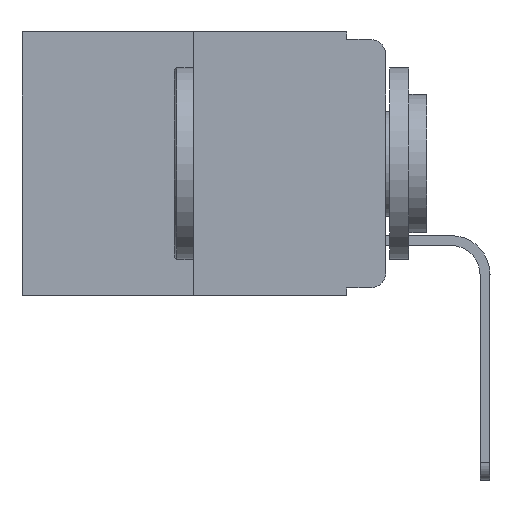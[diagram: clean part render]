
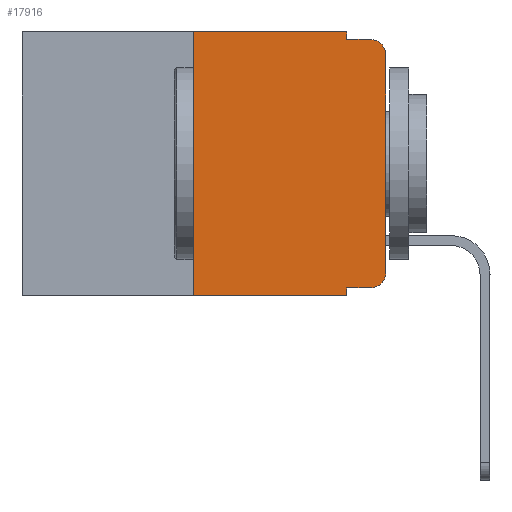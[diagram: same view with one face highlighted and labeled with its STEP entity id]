
A CAD part, left-side view. The second image highlights one B-rep face of the part: STEP entity #17916.
In plain terms, the highlighted planar face has unit normal (-1, 0, 0).
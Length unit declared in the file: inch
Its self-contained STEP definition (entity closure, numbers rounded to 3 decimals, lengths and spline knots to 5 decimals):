
#12 = CARTESIAN_POINT ( 'NONE',  ( 0., 0.051, 0. ) ) ;
#140 = DIRECTION ( 'NONE',  ( 1., 0., 0. ) ) ;
#257 = ORIENTED_EDGE ( 'NONE', *, *, #9310, .T. ) ;
#658 = EDGE_LOOP ( 'NONE', ( #20941, #257, #15732, #19808, #21544, #19864, #11440, #20858, #4094, #17182 ) ) ;
#941 = CIRCLE ( 'NONE', #20716, 0.02 ) ;
#1385 = CARTESIAN_POINT ( 'NONE',  ( 0., 0.25, 0. ) ) ;
#1411 = EDGE_CURVE ( 'NONE', #12307, #14423, #21536, .T. ) ;
#1836 = LINE ( 'NONE', #6421, #13147 ) ;
#2002 = CARTESIAN_POINT ( 'NONE',  ( 0., 0.051, 0. ) ) ;
#2283 = VERTEX_POINT ( 'NONE', #21336 ) ;
#2527 = VECTOR ( 'NONE', #4830, 39.37008 ) ;
#3348 = CARTESIAN_POINT ( 'NONE',  ( 0., 0., -0.03 ) ) ;
#3548 = VERTEX_POINT ( 'NONE', #5417 ) ;
#3852 = VERTEX_POINT ( 'NONE', #12 ) ;
#4060 = FACE_OUTER_BOUND ( 'NONE', #658, .T. ) ;
#4094 = ORIENTED_EDGE ( 'NONE', *, *, #9401, .T. ) ;
#4830 = DIRECTION ( 'NONE',  ( 0., -1., 0. ) ) ;
#5417 = CARTESIAN_POINT ( 'NONE',  ( 0., 0.051, -0.343 ) ) ;
#5623 = AXIS2_PLACEMENT_3D ( 'NONE', #18427, #140, #6646 ) ;
#5665 = CARTESIAN_POINT ( 'NONE',  ( 0., 0., -0.313 ) ) ;
#5753 = CIRCLE ( 'NONE', #15653, 0.02 ) ;
#6164 = VERTEX_POINT ( 'NONE', #5665 ) ;
#6421 = CARTESIAN_POINT ( 'NONE',  ( 0., 0., 0. ) ) ;
#6465 = VECTOR ( 'NONE', #10214, 39.37008 ) ;
#6640 = DIRECTION ( 'NONE',  ( 0., -1., 0. ) ) ;
#6646 = DIRECTION ( 'NONE',  ( 0., 0., -1. ) ) ;
#6752 = LINE ( 'NONE', #14120, #14620 ) ;
#6936 = VECTOR ( 'NONE', #6640, 39.37008 ) ;
#7056 = LINE ( 'NONE', #9909, #2527 ) ;
#8296 = LINE ( 'NONE', #2002, #6465 ) ;
#8330 = DIRECTION ( 'NONE',  ( 0., 0., -1. ) ) ;
#8343 = EDGE_CURVE ( 'NONE', #14423, #3852, #15329, .T. ) ;
#8749 = LINE ( 'NONE', #20451, #14000 ) ;
#8937 = EDGE_CURVE ( 'NONE', #2283, #6164, #5753, .T. ) ;
#9310 = EDGE_CURVE ( 'NONE', #11584, #20360, #941, .T. ) ;
#9401 = EDGE_CURVE ( 'NONE', #11858, #2283, #7056, .T. ) ;
#9909 = CARTESIAN_POINT ( 'NONE',  ( 0., 0.051, -0.333 ) ) ;
#9935 = EDGE_CURVE ( 'NONE', #11858, #3548, #6752, .T. ) ;
#9939 = DIRECTION ( 'NONE',  ( -1., 0., 0. ) ) ;
#10214 = DIRECTION ( 'NONE',  ( 0., 0., -1. ) ) ;
#11225 = DIRECTION ( 'NONE',  ( -1., 0., 0. ) ) ;
#11299 = DIRECTION ( 'NONE',  ( 0., 0., -1. ) ) ;
#11440 = ORIENTED_EDGE ( 'NONE', *, *, #19290, .T. ) ;
#11584 = VERTEX_POINT ( 'NONE', #3348 ) ;
#11618 = DIRECTION ( 'NONE',  ( 0., -1., 0. ) ) ;
#11858 = VERTEX_POINT ( 'NONE', #18894 ) ;
#12307 = VERTEX_POINT ( 'NONE', #18294 ) ;
#12654 = VECTOR ( 'NONE', #19732, 39.37008 ) ;
#12898 = VECTOR ( 'NONE', #11618, 39.37008 ) ;
#13147 = VECTOR ( 'NONE', #21284, 39.37008 ) ;
#13273 = CARTESIAN_POINT ( 'NONE',  ( 0., 0.02, -0.313 ) ) ;
#14000 = VECTOR ( 'NONE', #15491, 39.37008 ) ;
#14120 = CARTESIAN_POINT ( 'NONE',  ( 0., 0.051, 0. ) ) ;
#14346 = VERTEX_POINT ( 'NONE', #20467 ) ;
#14423 = VERTEX_POINT ( 'NONE', #20531 ) ;
#14562 = CARTESIAN_POINT ( 'NONE',  ( 0., 0.02, -0.01 ) ) ;
#14620 = VECTOR ( 'NONE', #8330, 39.37008 ) ;
#15016 = LINE ( 'NONE', #19559, #12898 ) ;
#15329 = LINE ( 'NONE', #16590, #6936 ) ;
#15491 = DIRECTION ( 'NONE',  ( 0., -1., 0. ) ) ;
#15653 = AXIS2_PLACEMENT_3D ( 'NONE', #13273, #9939, #18327 ) ;
#15732 = ORIENTED_EDGE ( 'NONE', *, *, #18688, .F. ) ;
#15970 = CARTESIAN_POINT ( 'NONE',  ( 0., 0.02, -0.03 ) ) ;
#16590 = CARTESIAN_POINT ( 'NONE',  ( 0., 0.473, 0. ) ) ;
#17182 = ORIENTED_EDGE ( 'NONE', *, *, #8937, .T. ) ;
#17324 = EDGE_CURVE ( 'NONE', #3852, #14346, #8296, .T. ) ;
#17916 = ADVANCED_FACE ( 'NONE', ( #4060 ), #20262, .F. ) ;
#18294 = CARTESIAN_POINT ( 'NONE',  ( 0., 0.25, -0.343 ) ) ;
#18327 = DIRECTION ( 'NONE',  ( 0., 0., -1. ) ) ;
#18427 = CARTESIAN_POINT ( 'NONE',  ( 0., 0.473, 0. ) ) ;
#18688 = EDGE_CURVE ( 'NONE', #14346, #20360, #8749, .T. ) ;
#18894 = CARTESIAN_POINT ( 'NONE',  ( 0., 0.051, -0.333 ) ) ;
#19290 = EDGE_CURVE ( 'NONE', #12307, #3548, #15016, .T. ) ;
#19559 = CARTESIAN_POINT ( 'NONE',  ( 0., 0.473, -0.343 ) ) ;
#19732 = DIRECTION ( 'NONE',  ( 0., 0., 1. ) ) ;
#19808 = ORIENTED_EDGE ( 'NONE', *, *, #17324, .F. ) ;
#19864 = ORIENTED_EDGE ( 'NONE', *, *, #1411, .F. ) ;
#20262 = PLANE ( 'NONE',  #5623 ) ;
#20360 = VERTEX_POINT ( 'NONE', #14562 ) ;
#20448 = EDGE_CURVE ( 'NONE', #6164, #11584, #1836, .T. ) ;
#20451 = CARTESIAN_POINT ( 'NONE',  ( 0., 0.051, -0.01 ) ) ;
#20467 = CARTESIAN_POINT ( 'NONE',  ( 0., 0.051, -0.01 ) ) ;
#20531 = CARTESIAN_POINT ( 'NONE',  ( 0., 0.25, 0. ) ) ;
#20716 = AXIS2_PLACEMENT_3D ( 'NONE', #15970, #11225, #11299 ) ;
#20858 = ORIENTED_EDGE ( 'NONE', *, *, #9935, .F. ) ;
#20941 = ORIENTED_EDGE ( 'NONE', *, *, #20448, .T. ) ;
#21284 = DIRECTION ( 'NONE',  ( 0., 0., 1. ) ) ;
#21336 = CARTESIAN_POINT ( 'NONE',  ( 0., 0.02, -0.333 ) ) ;
#21536 = LINE ( 'NONE', #1385, #12654 ) ;
#21544 = ORIENTED_EDGE ( 'NONE', *, *, #8343, .F. ) ;
